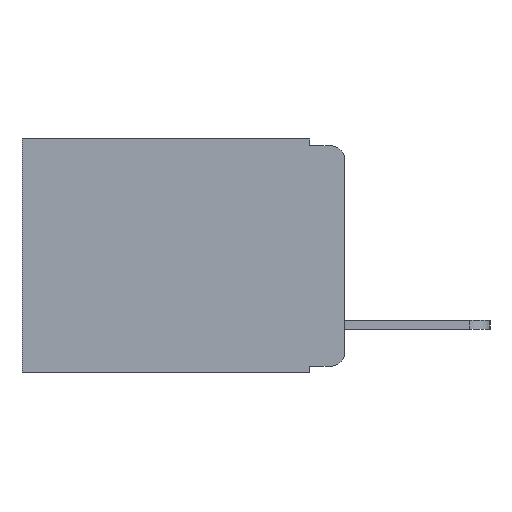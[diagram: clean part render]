
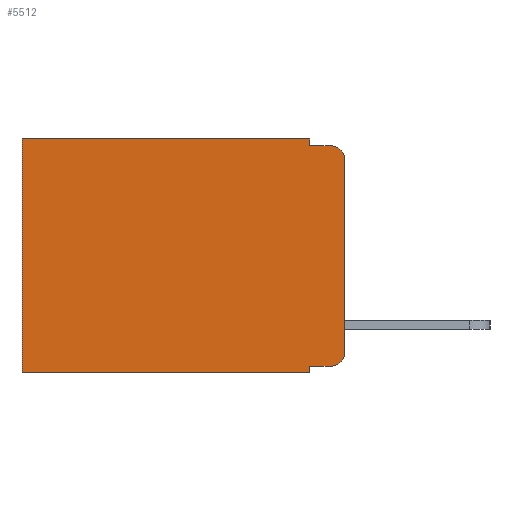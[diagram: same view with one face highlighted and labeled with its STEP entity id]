
A CAD part, left-side view. The second image highlights one B-rep face of the part: STEP entity #5512.
In plain terms, the highlighted planar face has unit normal (-1, 0, 0).
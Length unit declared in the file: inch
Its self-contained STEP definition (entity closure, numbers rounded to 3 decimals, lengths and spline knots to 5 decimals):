
#23 = DIRECTION ( 'NONE',  ( 1., 0., 0. ) ) ;
#80 = CARTESIAN_POINT ( 'NONE',  ( 0.298, 0.02, -0.313 ) ) ;
#136 = VECTOR ( 'NONE', #8643, 39.37008 ) ;
#619 = VERTEX_POINT ( 'NONE', #10187 ) ;
#737 = VECTOR ( 'NONE', #11723, 39.37008 ) ;
#800 = VERTEX_POINT ( 'NONE', #11816 ) ;
#1133 = EDGE_CURVE ( 'NONE', #1544, #6420, #10738, .T. ) ;
#1141 = CARTESIAN_POINT ( 'NONE',  ( 0.298, 0.473, 0. ) ) ;
#1269 = CARTESIAN_POINT ( 'NONE',  ( 0.298, 0.051, -0.343 ) ) ;
#1467 = LINE ( 'NONE', #6305, #6275 ) ;
#1470 = DIRECTION ( 'NONE',  ( 0., 0., -1. ) ) ;
#1544 = VERTEX_POINT ( 'NONE', #9596 ) ;
#1788 = DIRECTION ( 'NONE',  ( 0., 0., -1. ) ) ;
#1858 = CIRCLE ( 'NONE', #2177, 0.02 ) ;
#1944 = ORIENTED_EDGE ( 'NONE', *, *, #9809, .T. ) ;
#2074 = LINE ( 'NONE', #1141, #737 ) ;
#2168 = AXIS2_PLACEMENT_3D ( 'NONE', #2345, #23, #9192 ) ;
#2177 = AXIS2_PLACEMENT_3D ( 'NONE', #11058, #7909, #8797 ) ;
#2291 = ORIENTED_EDGE ( 'NONE', *, *, #11294, .F. ) ;
#2324 = CARTESIAN_POINT ( 'NONE',  ( 0.298, 0.051, -0.333 ) ) ;
#2345 = CARTESIAN_POINT ( 'NONE',  ( 0.298, 0., 0. ) ) ;
#2356 = CARTESIAN_POINT ( 'NONE',  ( 0.298, 0.051, 0. ) ) ;
#2604 = EDGE_CURVE ( 'NONE', #7479, #8937, #8761, .T. ) ;
#3303 = ORIENTED_EDGE ( 'NONE', *, *, #2604, .T. ) ;
#3383 = LINE ( 'NONE', #6107, #5156 ) ;
#3536 = ORIENTED_EDGE ( 'NONE', *, *, #5336, .F. ) ;
#3827 = CIRCLE ( 'NONE', #6665, 0.02 ) ;
#4106 = DIRECTION ( 'NONE',  ( 0., -1., 0. ) ) ;
#4114 = CARTESIAN_POINT ( 'NONE',  ( 0.298, 0.051, -0.333 ) ) ;
#4131 = VECTOR ( 'NONE', #6628, 39.37008 ) ;
#4435 = VERTEX_POINT ( 'NONE', #5807 ) ;
#4447 = LINE ( 'NONE', #7745, #136 ) ;
#4712 = EDGE_LOOP ( 'NONE', ( #10284, #1944, #3536, #12029, #3303, #4968, #2291, #7076, #6061, #10315 ) ) ;
#4841 = EDGE_CURVE ( 'NONE', #8537, #4435, #5282, .T. ) ;
#4968 = ORIENTED_EDGE ( 'NONE', *, *, #6866, .T. ) ;
#5069 = EDGE_CURVE ( 'NONE', #4435, #6420, #3827, .T. ) ;
#5156 = VECTOR ( 'NONE', #7095, 39.37008 ) ;
#5279 = VERTEX_POINT ( 'NONE', #6807 ) ;
#5282 = LINE ( 'NONE', #4114, #11527 ) ;
#5336 = EDGE_CURVE ( 'NONE', #800, #619, #4447, .T. ) ;
#5512 = ADVANCED_FACE ( 'NONE', ( #7834 ), #12016, .F. ) ;
#5571 = DIRECTION ( 'NONE',  ( -1., 0., 0. ) ) ;
#5807 = CARTESIAN_POINT ( 'NONE',  ( 0.298, 0.02, -0.333 ) ) ;
#5918 = EDGE_CURVE ( 'NONE', #8537, #8951, #3383, .T. ) ;
#6061 = ORIENTED_EDGE ( 'NONE', *, *, #4841, .T. ) ;
#6107 = CARTESIAN_POINT ( 'NONE',  ( 0.298, 0.051, 0. ) ) ;
#6275 = VECTOR ( 'NONE', #8283, 39.37008 ) ;
#6305 = CARTESIAN_POINT ( 'NONE',  ( 0.298, 0., -0.343 ) ) ;
#6420 = VERTEX_POINT ( 'NONE', #8312 ) ;
#6628 = DIRECTION ( 'NONE',  ( 0., 0., -1. ) ) ;
#6665 = AXIS2_PLACEMENT_3D ( 'NONE', #80, #5571, #1470 ) ;
#6807 = CARTESIAN_POINT ( 'NONE',  ( 0.298, 0.473, -0.343 ) ) ;
#6866 = EDGE_CURVE ( 'NONE', #8937, #5279, #2074, .T. ) ;
#7076 = ORIENTED_EDGE ( 'NONE', *, *, #5918, .F. ) ;
#7095 = DIRECTION ( 'NONE',  ( 0., 0., -1. ) ) ;
#7112 = EDGE_CURVE ( 'NONE', #7479, #800, #10344, .T. ) ;
#7479 = VERTEX_POINT ( 'NONE', #2356 ) ;
#7745 = CARTESIAN_POINT ( 'NONE',  ( 0.298, 0.051, -0.01 ) ) ;
#7834 = FACE_OUTER_BOUND ( 'NONE', #4712, .T. ) ;
#7839 = VECTOR ( 'NONE', #1788, 39.37008 ) ;
#7909 = DIRECTION ( 'NONE',  ( -1., 0., 0. ) ) ;
#8283 = DIRECTION ( 'NONE',  ( 0., 1., 0. ) ) ;
#8312 = CARTESIAN_POINT ( 'NONE',  ( 0.298, 0., -0.313 ) ) ;
#8537 = VERTEX_POINT ( 'NONE', #2324 ) ;
#8622 = VECTOR ( 'NONE', #9421, 39.37008 ) ;
#8643 = DIRECTION ( 'NONE',  ( 0., -1., 0. ) ) ;
#8761 = LINE ( 'NONE', #9474, #8622 ) ;
#8797 = DIRECTION ( 'NONE',  ( 0., 0., -1. ) ) ;
#8937 = VERTEX_POINT ( 'NONE', #11096 ) ;
#8951 = VERTEX_POINT ( 'NONE', #1269 ) ;
#9192 = DIRECTION ( 'NONE',  ( 0., 0., -1. ) ) ;
#9252 = CARTESIAN_POINT ( 'NONE',  ( 0.298, 0., 0. ) ) ;
#9421 = DIRECTION ( 'NONE',  ( 0., 1., 0. ) ) ;
#9474 = CARTESIAN_POINT ( 'NONE',  ( 0.298, 0., 0. ) ) ;
#9596 = CARTESIAN_POINT ( 'NONE',  ( 0.298, 0., -0.03 ) ) ;
#9809 = EDGE_CURVE ( 'NONE', #1544, #619, #1858, .T. ) ;
#10187 = CARTESIAN_POINT ( 'NONE',  ( 0.298, 0.02, -0.01 ) ) ;
#10284 = ORIENTED_EDGE ( 'NONE', *, *, #1133, .F. ) ;
#10315 = ORIENTED_EDGE ( 'NONE', *, *, #5069, .T. ) ;
#10344 = LINE ( 'NONE', #10399, #4131 ) ;
#10399 = CARTESIAN_POINT ( 'NONE',  ( 0.298, 0.051, 0. ) ) ;
#10738 = LINE ( 'NONE', #9252, #7839 ) ;
#11058 = CARTESIAN_POINT ( 'NONE',  ( 0.298, 0.02, -0.03 ) ) ;
#11096 = CARTESIAN_POINT ( 'NONE',  ( 0.298, 0.473, 0. ) ) ;
#11294 = EDGE_CURVE ( 'NONE', #8951, #5279, #1467, .T. ) ;
#11527 = VECTOR ( 'NONE', #4106, 39.37008 ) ;
#11723 = DIRECTION ( 'NONE',  ( 0., 0., -1. ) ) ;
#11816 = CARTESIAN_POINT ( 'NONE',  ( 0.298, 0.051, -0.01 ) ) ;
#12016 = PLANE ( 'NONE',  #2168 ) ;
#12029 = ORIENTED_EDGE ( 'NONE', *, *, #7112, .F. ) ;
